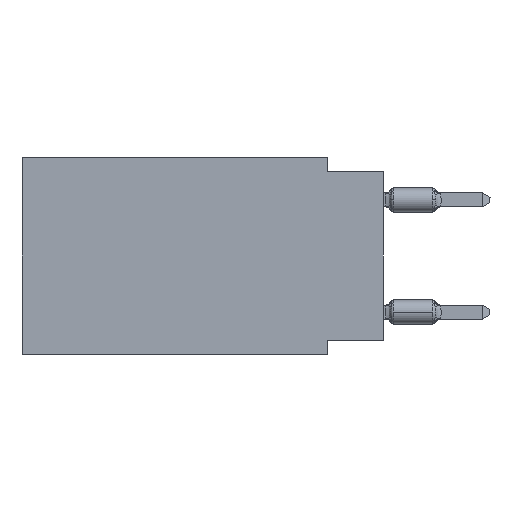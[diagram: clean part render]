
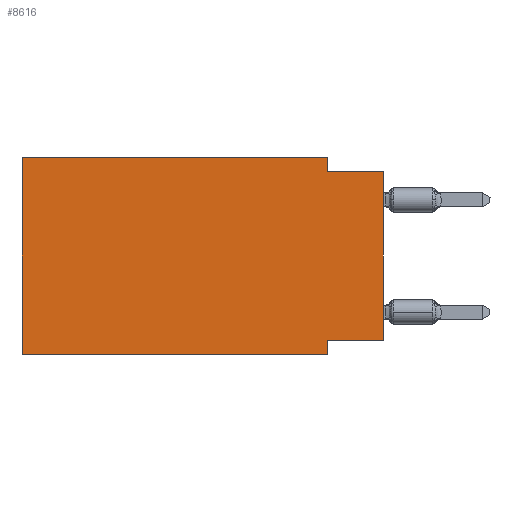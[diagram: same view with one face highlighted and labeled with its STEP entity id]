
A CAD part, left-side view. The second image highlights one B-rep face of the part: STEP entity #8616.
In plain terms, the highlighted planar face has unit normal (-1, 0, 0).
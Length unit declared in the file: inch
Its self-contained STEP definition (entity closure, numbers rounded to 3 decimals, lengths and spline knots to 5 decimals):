
#319 = EDGE_CURVE ( 'NONE', #8631, #20457, #24812, .T. ) ;
#772 = CARTESIAN_POINT ( 'NONE',  ( 0., 0.1, -0.35 ) ) ;
#840 = EDGE_CURVE ( 'NONE', #10574, #32457, #9640, .T. ) ;
#1010 = DIRECTION ( 'NONE',  ( 1., 0., 0. ) ) ;
#1285 = ORIENTED_EDGE ( 'NONE', *, *, #840, .F. ) ;
#2084 = CARTESIAN_POINT ( 'NONE',  ( 0., 0., -0.025 ) ) ;
#2751 = LINE ( 'NONE', #772, #3825 ) ;
#3406 = ORIENTED_EDGE ( 'NONE', *, *, #18142, .F. ) ;
#3782 = CARTESIAN_POINT ( 'NONE',  ( 0., 0.645, 0. ) ) ;
#3825 = VECTOR ( 'NONE', #15427, 39.37008 ) ;
#4085 = ORIENTED_EDGE ( 'NONE', *, *, #13666, .T. ) ;
#4367 = VECTOR ( 'NONE', #23458, 39.37008 ) ;
#4884 = DIRECTION ( 'NONE',  ( 0., 0., -1. ) ) ;
#6173 = DIRECTION ( 'NONE',  ( 0., 1., 0. ) ) ;
#6496 = CARTESIAN_POINT ( 'NONE',  ( 0., 0., -0.325 ) ) ;
#7656 = EDGE_CURVE ( 'NONE', #30338, #27705, #2751, .T. ) ;
#8149 = EDGE_CURVE ( 'NONE', #10574, #27705, #10457, .T. ) ;
#8163 = DIRECTION ( 'NONE',  ( 0., -1., 0. ) ) ;
#8228 = EDGE_CURVE ( 'NONE', #32457, #8631, #8654, .T. ) ;
#8290 = EDGE_CURVE ( 'NONE', #11189, #30338, #19007, .T. ) ;
#8616 = ADVANCED_FACE ( 'NONE', ( #11255 ), #31518, .F. ) ;
#8631 = VERTEX_POINT ( 'NONE', #18970 ) ;
#8654 = LINE ( 'NONE', #19172, #4367 ) ;
#9640 = LINE ( 'NONE', #28066, #9967 ) ;
#9817 = VECTOR ( 'NONE', #28084, 39.37008 ) ;
#9967 = VECTOR ( 'NONE', #32550, 39.37008 ) ;
#10457 = LINE ( 'NONE', #20349, #32284 ) ;
#10574 = VERTEX_POINT ( 'NONE', #21666 ) ;
#10747 = CARTESIAN_POINT ( 'NONE',  ( 0., 0., -0.325 ) ) ;
#11189 = VERTEX_POINT ( 'NONE', #10747 ) ;
#11255 = FACE_OUTER_BOUND ( 'NONE', #27494, .T. ) ;
#11454 = VERTEX_POINT ( 'NONE', #19612 ) ;
#12801 = VECTOR ( 'NONE', #6173, 39.37008 ) ;
#13666 = EDGE_CURVE ( 'NONE', #11189, #11454, #26263, .T. ) ;
#14767 = VECTOR ( 'NONE', #26985, 39.37008 ) ;
#15427 = DIRECTION ( 'NONE',  ( 0., 0., -1. ) ) ;
#18039 = CARTESIAN_POINT ( 'NONE',  ( 0., 0., 0. ) ) ;
#18142 = EDGE_CURVE ( 'NONE', #20457, #11454, #27474, .T. ) ;
#18322 = CARTESIAN_POINT ( 'NONE',  ( 0., 0.645, 0. ) ) ;
#18970 = CARTESIAN_POINT ( 'NONE',  ( 0., 0.1, 0. ) ) ;
#19007 = LINE ( 'NONE', #6496, #12801 ) ;
#19172 = CARTESIAN_POINT ( 'NONE',  ( 0., 0.645, 0. ) ) ;
#19612 = CARTESIAN_POINT ( 'NONE',  ( 0., 0., -0.025 ) ) ;
#20349 = CARTESIAN_POINT ( 'NONE',  ( 0., 0.645, -0.35 ) ) ;
#20457 = VERTEX_POINT ( 'NONE', #32130 ) ;
#21376 = ORIENTED_EDGE ( 'NONE', *, *, #8149, .T. ) ;
#21666 = CARTESIAN_POINT ( 'NONE',  ( 0., 0.645, -0.35 ) ) ;
#21728 = ORIENTED_EDGE ( 'NONE', *, *, #8290, .F. ) ;
#23458 = DIRECTION ( 'NONE',  ( 0., -1., 0. ) ) ;
#24028 = CARTESIAN_POINT ( 'NONE',  ( 0., 0.1, -0.35 ) ) ;
#24446 = CARTESIAN_POINT ( 'NONE',  ( 0., 0.1, -0.325 ) ) ;
#24812 = LINE ( 'NONE', #29609, #30782 ) ;
#26263 = LINE ( 'NONE', #18039, #9817 ) ;
#26985 = DIRECTION ( 'NONE',  ( 0., -1., 0. ) ) ;
#27474 = LINE ( 'NONE', #2084, #14767 ) ;
#27494 = EDGE_LOOP ( 'NONE', ( #4085, #3406, #28473, #32151, #1285, #21376, #27821, #21728 ) ) ;
#27705 = VERTEX_POINT ( 'NONE', #24028 ) ;
#27821 = ORIENTED_EDGE ( 'NONE', *, *, #7656, .F. ) ;
#28066 = CARTESIAN_POINT ( 'NONE',  ( 0., 0.645, 0. ) ) ;
#28084 = DIRECTION ( 'NONE',  ( 0., 0., 1. ) ) ;
#28473 = ORIENTED_EDGE ( 'NONE', *, *, #319, .F. ) ;
#29609 = CARTESIAN_POINT ( 'NONE',  ( 0., 0.1, 0. ) ) ;
#30338 = VERTEX_POINT ( 'NONE', #24446 ) ;
#30782 = VECTOR ( 'NONE', #4884, 39.37008 ) ;
#31024 = DIRECTION ( 'NONE',  ( 0., 0., -1. ) ) ;
#31518 = PLANE ( 'NONE',  #32314 ) ;
#32130 = CARTESIAN_POINT ( 'NONE',  ( 0., 0.1, -0.025 ) ) ;
#32151 = ORIENTED_EDGE ( 'NONE', *, *, #8228, .F. ) ;
#32284 = VECTOR ( 'NONE', #8163, 39.37008 ) ;
#32314 = AXIS2_PLACEMENT_3D ( 'NONE', #18322, #1010, #31024 ) ;
#32457 = VERTEX_POINT ( 'NONE', #3782 ) ;
#32550 = DIRECTION ( 'NONE',  ( 0., 0., 1. ) ) ;
